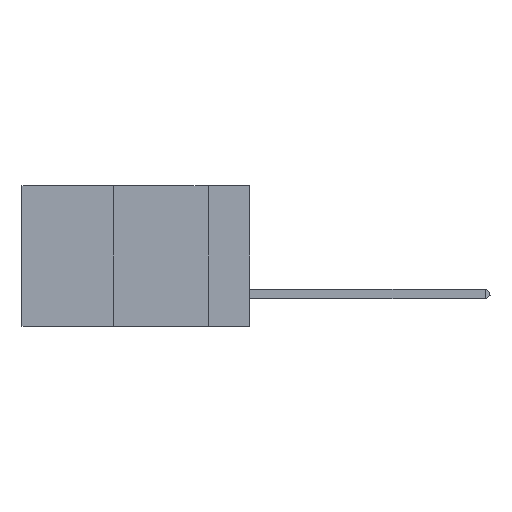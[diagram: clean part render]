
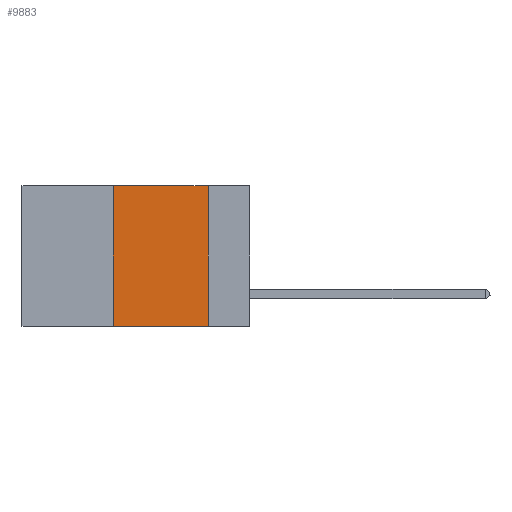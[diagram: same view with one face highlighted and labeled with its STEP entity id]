
A CAD part, left-side view. The second image highlights one B-rep face of the part: STEP entity #9883.
In plain terms, the highlighted planar face has unit normal (-1, 0, 0).
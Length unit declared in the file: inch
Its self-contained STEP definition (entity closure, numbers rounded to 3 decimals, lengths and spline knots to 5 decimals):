
#38 = EDGE_CURVE ( 'NONE', #1407, #12106, #6616, .T. ) ;
#517 = CARTESIAN_POINT ( 'NONE',  ( 0., 0.36, -0.37 ) ) ;
#629 = LINE ( 'NONE', #11461, #1093 ) ;
#726 = VECTOR ( 'NONE', #2468, 39.37008 ) ;
#1093 = VECTOR ( 'NONE', #12399, 39.37008 ) ;
#1407 = VERTEX_POINT ( 'NONE', #517 ) ;
#2468 = DIRECTION ( 'NONE',  ( 0., 0., 1. ) ) ;
#3235 = ORIENTED_EDGE ( 'NONE', *, *, #12198, .F. ) ;
#3321 = EDGE_LOOP ( 'NONE', ( #10712, #11549, #3235, #6130 ) ) ;
#3761 = LINE ( 'NONE', #4182, #726 ) ;
#4182 = CARTESIAN_POINT ( 'NONE',  ( 0., 0.36, 0. ) ) ;
#4513 = EDGE_CURVE ( 'NONE', #13076, #6921, #12981, .T. ) ;
#5116 = CARTESIAN_POINT ( 'NONE',  ( 0., 0.36, 0. ) ) ;
#5558 = DIRECTION ( 'NONE',  ( 0., -1., 0. ) ) ;
#5660 = AXIS2_PLACEMENT_3D ( 'NONE', #11177, #9064, #7022 ) ;
#6062 = CARTESIAN_POINT ( 'NONE',  ( 0., 0.11, 0. ) ) ;
#6130 = ORIENTED_EDGE ( 'NONE', *, *, #38, .T. ) ;
#6239 = VECTOR ( 'NONE', #6261, 39.37008 ) ;
#6261 = DIRECTION ( 'NONE',  ( 0., -1., 0. ) ) ;
#6616 = LINE ( 'NONE', #10080, #11760 ) ;
#6921 = VERTEX_POINT ( 'NONE', #6062 ) ;
#7022 = DIRECTION ( 'NONE',  ( 0., 0., -1. ) ) ;
#8093 = PLANE ( 'NONE',  #5660 ) ;
#8304 = CARTESIAN_POINT ( 'NONE',  ( 0., 0.11, -0.37 ) ) ;
#9064 = DIRECTION ( 'NONE',  ( 1., 0., 0. ) ) ;
#9330 = EDGE_CURVE ( 'NONE', #6921, #12106, #629, .T. ) ;
#9883 = ADVANCED_FACE ( 'NONE', ( #11671 ), #8093, .F. ) ;
#10080 = CARTESIAN_POINT ( 'NONE',  ( 0., 0.6, -0.37 ) ) ;
#10712 = ORIENTED_EDGE ( 'NONE', *, *, #9330, .F. ) ;
#11177 = CARTESIAN_POINT ( 'NONE',  ( 0., 0.6, 0. ) ) ;
#11461 = CARTESIAN_POINT ( 'NONE',  ( 0., 0.11, 0. ) ) ;
#11549 = ORIENTED_EDGE ( 'NONE', *, *, #4513, .F. ) ;
#11671 = FACE_OUTER_BOUND ( 'NONE', #3321, .T. ) ;
#11760 = VECTOR ( 'NONE', #5558, 39.37008 ) ;
#12106 = VERTEX_POINT ( 'NONE', #8304 ) ;
#12198 = EDGE_CURVE ( 'NONE', #1407, #13076, #3761, .T. ) ;
#12302 = CARTESIAN_POINT ( 'NONE',  ( 0., 0.6, 0. ) ) ;
#12399 = DIRECTION ( 'NONE',  ( 0., 0., -1. ) ) ;
#12981 = LINE ( 'NONE', #12302, #6239 ) ;
#13076 = VERTEX_POINT ( 'NONE', #5116 ) ;
